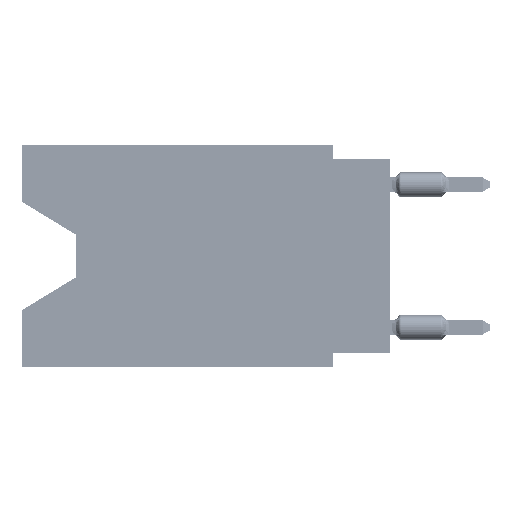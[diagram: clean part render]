
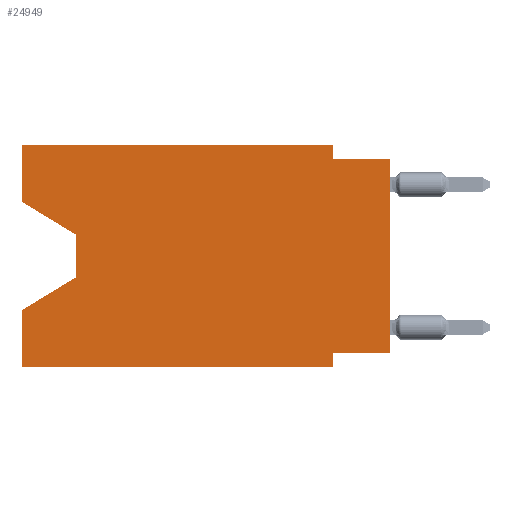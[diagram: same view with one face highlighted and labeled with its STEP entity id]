
A CAD part, left-side view. The second image highlights one B-rep face of the part: STEP entity #24949.
In plain terms, the highlighted planar face has unit normal (-1, 0, 0).
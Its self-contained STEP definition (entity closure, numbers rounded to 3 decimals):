
#295 = DIRECTION ( 'NONE',  ( 0., 0., 1. ) ) ;
#832 = DIRECTION ( 'NONE',  ( 1., 0., 0. ) ) ;
#1201 = LINE ( 'NONE', #2394, #4045 ) ;
#1209 = ORIENTED_EDGE ( 'NONE', *, *, #56767, .T. ) ;
#1773 = LINE ( 'NONE', #46126, #35684 ) ;
#2316 = VERTEX_POINT ( 'NONE', #2525 ) ;
#2317 = VECTOR ( 'NONE', #8404, 1000. ) ;
#2394 = CARTESIAN_POINT ( 'NONE',  ( 0., 16.383, -2.546 ) ) ;
#2525 = CARTESIAN_POINT ( 'NONE',  ( 0., 2.54, -9.271 ) ) ;
#2918 = VERTEX_POINT ( 'NONE', #16658 ) ;
#3085 = LINE ( 'NONE', #71872, #2317 ) ;
#3674 = ORIENTED_EDGE ( 'NONE', *, *, #74731, .T. ) ;
#4045 = VECTOR ( 'NONE', #50055, 1000. ) ;
#5748 = PLANE ( 'NONE',  #27960 ) ;
#6930 = VERTEX_POINT ( 'NONE', #75262 ) ;
#7379 = EDGE_CURVE ( 'NONE', #56487, #2316, #20219, .T. ) ;
#8404 = DIRECTION ( 'NONE',  ( 0., -1., 0. ) ) ;
#8999 = CARTESIAN_POINT ( 'NONE',  ( 0., 16.383, 0. ) ) ;
#9465 = VERTEX_POINT ( 'NONE', #65948 ) ;
#9614 = LINE ( 'NONE', #79571, #20646 ) ;
#10386 = VERTEX_POINT ( 'NONE', #69373 ) ;
#10403 = EDGE_CURVE ( 'NONE', #9465, #14682, #61665, .T. ) ;
#10792 = DIRECTION ( 'NONE',  ( 0., -1., 0. ) ) ;
#11922 = VECTOR ( 'NONE', #295, 1000. ) ;
#13420 = CARTESIAN_POINT ( 'NONE',  ( 0., 16.383, -2.546 ) ) ;
#13611 = LINE ( 'NONE', #70154, #21559 ) ;
#13985 = EDGE_CURVE ( 'NONE', #19372, #10386, #3085, .T. ) ;
#14682 = VERTEX_POINT ( 'NONE', #61139 ) ;
#15639 = VERTEX_POINT ( 'NONE', #44229 ) ;
#16658 = CARTESIAN_POINT ( 'NONE',  ( 0., 13.97, -5.893 ) ) ;
#18109 = VECTOR ( 'NONE', #72458, 1000. ) ;
#18626 = CARTESIAN_POINT ( 'NONE',  ( 0., 0., -9.271 ) ) ;
#19372 = VERTEX_POINT ( 'NONE', #33490 ) ;
#19621 = DIRECTION ( 'NONE',  ( 0., 0., -1. ) ) ;
#19841 = ORIENTED_EDGE ( 'NONE', *, *, #40307, .F. ) ;
#20057 = VECTOR ( 'NONE', #70656, 1000. ) ;
#20219 = LINE ( 'NONE', #64557, #20057 ) ;
#20392 = EDGE_CURVE ( 'NONE', #2918, #14682, #37489, .T. ) ;
#20646 = VECTOR ( 'NONE', #43655, 1000. ) ;
#21559 = VECTOR ( 'NONE', #50238, 1000. ) ;
#24102 = VERTEX_POINT ( 'NONE', #49795 ) ;
#24745 = LINE ( 'NONE', #49555, #11922 ) ;
#24949 = ADVANCED_FACE ( 'NONE', ( #38274 ), #5748, .F. ) ;
#25284 = CARTESIAN_POINT ( 'NONE',  ( 0., 13.97, -5.893 ) ) ;
#25682 = DIRECTION ( 'NONE',  ( 0., 0., -1. ) ) ;
#27960 = AXIS2_PLACEMENT_3D ( 'NONE', #50078, #832, #25682 ) ;
#31558 = CARTESIAN_POINT ( 'NONE',  ( 0., 16.383, 0. ) ) ;
#32176 = EDGE_CURVE ( 'NONE', #56487, #24102, #24745, .T. ) ;
#33490 = CARTESIAN_POINT ( 'NONE',  ( 0., 16.383, 0. ) ) ;
#35684 = VECTOR ( 'NONE', #70952, 1000. ) ;
#37489 = LINE ( 'NONE', #25284, #73014 ) ;
#38213 = ORIENTED_EDGE ( 'NONE', *, *, #7379, .F. ) ;
#38274 = FACE_OUTER_BOUND ( 'NONE', #60794, .T. ) ;
#40307 = EDGE_CURVE ( 'NONE', #6930, #24102, #46221, .T. ) ;
#41131 = LINE ( 'NONE', #8999, #18109 ) ;
#42858 = EDGE_CURVE ( 'NONE', #2316, #15639, #13611, .T. ) ;
#43421 = ORIENTED_EDGE ( 'NONE', *, *, #58616, .T. ) ;
#43655 = DIRECTION ( 'NONE',  ( 0., -1., 0. ) ) ;
#43885 = ORIENTED_EDGE ( 'NONE', *, *, #42858, .F. ) ;
#44229 = CARTESIAN_POINT ( 'NONE',  ( 0., 2.54, -9.906 ) ) ;
#46126 = CARTESIAN_POINT ( 'NONE',  ( 0., 2.54, 0. ) ) ;
#46221 = LINE ( 'NONE', #72632, #78859 ) ;
#49555 = CARTESIAN_POINT ( 'NONE',  ( 0., 0., 0. ) ) ;
#49795 = CARTESIAN_POINT ( 'NONE',  ( 0., 0., -0.635 ) ) ;
#50055 = DIRECTION ( 'NONE',  ( 0., -0.855, -0.519 ) ) ;
#50078 = CARTESIAN_POINT ( 'NONE',  ( 0., 16.383, 0. ) ) ;
#50238 = DIRECTION ( 'NONE',  ( 0., 0., -1. ) ) ;
#50936 = LINE ( 'NONE', #75756, #71292 ) ;
#55307 = EDGE_CURVE ( 'NONE', #10386, #6930, #1773, .T. ) ;
#55457 = ORIENTED_EDGE ( 'NONE', *, *, #20392, .T. ) ;
#56487 = VERTEX_POINT ( 'NONE', #18626 ) ;
#56767 = EDGE_CURVE ( 'NONE', #9465, #15639, #9614, .T. ) ;
#58005 = ORIENTED_EDGE ( 'NONE', *, *, #58823, .F. ) ;
#58395 = ORIENTED_EDGE ( 'NONE', *, *, #13985, .F. ) ;
#58616 = EDGE_CURVE ( 'NONE', #67018, #2918, #50936, .T. ) ;
#58823 = EDGE_CURVE ( 'NONE', #60399, #19372, #41131, .T. ) ;
#58982 = ORIENTED_EDGE ( 'NONE', *, *, #55307, .F. ) ;
#60399 = VERTEX_POINT ( 'NONE', #13420 ) ;
#60588 = VECTOR ( 'NONE', #68166, 1000. ) ;
#60794 = EDGE_LOOP ( 'NONE', ( #3674, #43421, #55457, #71484, #1209, #43885, #38213, #73818, #19841, #58982, #58395, #58005 ) ) ;
#61139 = CARTESIAN_POINT ( 'NONE',  ( 0., 16.383, -7.36 ) ) ;
#61665 = LINE ( 'NONE', #31558, #60588 ) ;
#64557 = CARTESIAN_POINT ( 'NONE',  ( 0., 0., -9.271 ) ) ;
#65948 = CARTESIAN_POINT ( 'NONE',  ( 0., 16.383, -9.906 ) ) ;
#67018 = VERTEX_POINT ( 'NONE', #77114 ) ;
#68166 = DIRECTION ( 'NONE',  ( 0., 0., 1. ) ) ;
#69210 = DIRECTION ( 'NONE',  ( 0., 0.855, -0.519 ) ) ;
#69373 = CARTESIAN_POINT ( 'NONE',  ( 0., 2.54, 0. ) ) ;
#70154 = CARTESIAN_POINT ( 'NONE',  ( 0., 2.54, -9.906 ) ) ;
#70656 = DIRECTION ( 'NONE',  ( 0., 1., 0. ) ) ;
#70952 = DIRECTION ( 'NONE',  ( 0., 0., -1. ) ) ;
#71292 = VECTOR ( 'NONE', #19621, 1000. ) ;
#71484 = ORIENTED_EDGE ( 'NONE', *, *, #10403, .F. ) ;
#71872 = CARTESIAN_POINT ( 'NONE',  ( 0., 16.383, 0. ) ) ;
#72458 = DIRECTION ( 'NONE',  ( 0., 0., 1. ) ) ;
#72632 = CARTESIAN_POINT ( 'NONE',  ( 0., 0., -0.635 ) ) ;
#73014 = VECTOR ( 'NONE', #69210, 1000. ) ;
#73818 = ORIENTED_EDGE ( 'NONE', *, *, #32176, .T. ) ;
#74731 = EDGE_CURVE ( 'NONE', #60399, #67018, #1201, .T. ) ;
#75262 = CARTESIAN_POINT ( 'NONE',  ( 0., 2.54, -0.635 ) ) ;
#75756 = CARTESIAN_POINT ( 'NONE',  ( 0., 13.97, -4.013 ) ) ;
#77114 = CARTESIAN_POINT ( 'NONE',  ( 0., 13.97, -4.013 ) ) ;
#78859 = VECTOR ( 'NONE', #10792, 1000. ) ;
#79571 = CARTESIAN_POINT ( 'NONE',  ( 0., 16.383, -9.906 ) ) ;
